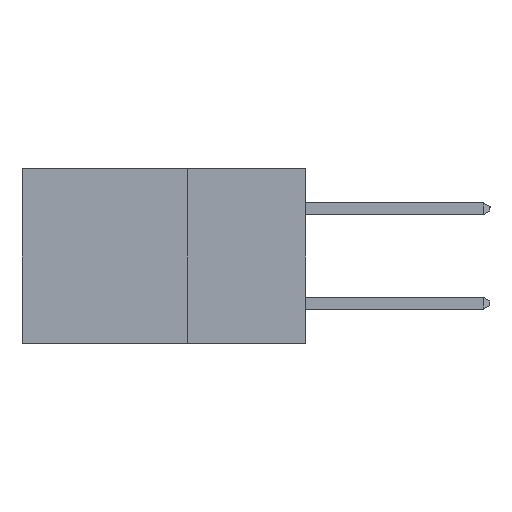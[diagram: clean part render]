
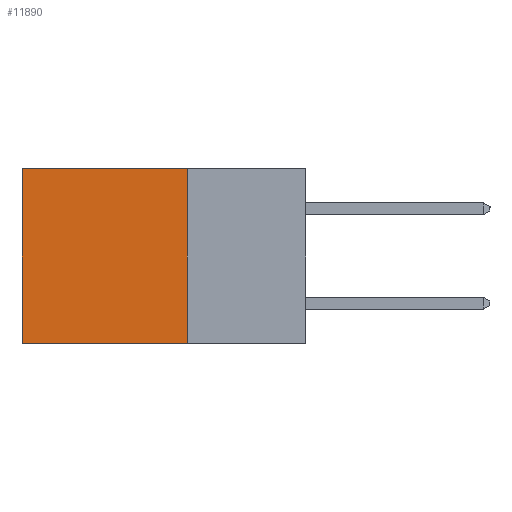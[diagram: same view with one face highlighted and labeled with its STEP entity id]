
A CAD part, left-side view. The second image highlights one B-rep face of the part: STEP entity #11890.
In plain terms, the highlighted planar face has unit normal (-1, 0, 0).
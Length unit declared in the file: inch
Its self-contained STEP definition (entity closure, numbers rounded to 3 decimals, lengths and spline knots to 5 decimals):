
#91 = FACE_OUTER_BOUND ( 'NONE', #2396, .T. ) ;
#130 = VERTEX_POINT ( 'NONE', #3008 ) ;
#530 = VECTOR ( 'NONE', #5643, 39.37008 ) ;
#1620 = EDGE_CURVE ( 'NONE', #5741, #1765, #5937, .T. ) ;
#1765 = VERTEX_POINT ( 'NONE', #3293 ) ;
#2021 = DIRECTION ( 'NONE',  ( 1., 0., 0. ) ) ;
#2396 = EDGE_LOOP ( 'NONE', ( #10595, #7719, #10690, #7004 ) ) ;
#2442 = CARTESIAN_POINT ( 'NONE',  ( 0.2615, 0.25, 0. ) ) ;
#2976 = PLANE ( 'NONE',  #8566 ) ;
#3008 = CARTESIAN_POINT ( 'NONE',  ( 0.2615, 0.6, -0.37 ) ) ;
#3220 = EDGE_CURVE ( 'NONE', #5741, #6571, #9048, .T. ) ;
#3290 = EDGE_CURVE ( 'NONE', #1765, #130, #4411, .T. ) ;
#3293 = CARTESIAN_POINT ( 'NONE',  ( 0.2615, 0.25, -0.37 ) ) ;
#3330 = CARTESIAN_POINT ( 'NONE',  ( 0.2615, 0.25, -0.37 ) ) ;
#3686 = CARTESIAN_POINT ( 'NONE',  ( 0.2615, 0.6, 0. ) ) ;
#3699 = CARTESIAN_POINT ( 'NONE',  ( 0.2615, 0.6, -0.37 ) ) ;
#3981 = DIRECTION ( 'NONE',  ( 0., 0., -1. ) ) ;
#4033 = VECTOR ( 'NONE', #10693, 39.37008 ) ;
#4410 = VECTOR ( 'NONE', #5006, 39.37008 ) ;
#4411 = LINE ( 'NONE', #3330, #9149 ) ;
#4954 = EDGE_CURVE ( 'NONE', #6571, #130, #9843, .T. ) ;
#5006 = DIRECTION ( 'NONE',  ( 0., 1., 0. ) ) ;
#5643 = DIRECTION ( 'NONE',  ( 0., 0., -1. ) ) ;
#5741 = VERTEX_POINT ( 'NONE', #2442 ) ;
#5937 = LINE ( 'NONE', #7801, #4033 ) ;
#6571 = VERTEX_POINT ( 'NONE', #3686 ) ;
#6877 = CARTESIAN_POINT ( 'NONE',  ( 0.2615, 0.25, -0.37 ) ) ;
#7004 = ORIENTED_EDGE ( 'NONE', *, *, #3220, .T. ) ;
#7719 = ORIENTED_EDGE ( 'NONE', *, *, #3290, .F. ) ;
#7801 = CARTESIAN_POINT ( 'NONE',  ( 0.2615, 0.25, -0.37 ) ) ;
#8566 = AXIS2_PLACEMENT_3D ( 'NONE', #6877, #2021, #3981 ) ;
#9048 = LINE ( 'NONE', #9895, #4410 ) ;
#9149 = VECTOR ( 'NONE', #10211, 39.37008 ) ;
#9843 = LINE ( 'NONE', #3699, #530 ) ;
#9895 = CARTESIAN_POINT ( 'NONE',  ( 0.2615, 0.25, 0. ) ) ;
#10211 = DIRECTION ( 'NONE',  ( 0., 1., 0. ) ) ;
#10595 = ORIENTED_EDGE ( 'NONE', *, *, #4954, .T. ) ;
#10690 = ORIENTED_EDGE ( 'NONE', *, *, #1620, .F. ) ;
#10693 = DIRECTION ( 'NONE',  ( 0., 0., -1. ) ) ;
#11890 = ADVANCED_FACE ( 'NONE', ( #91 ), #2976, .F. ) ;
